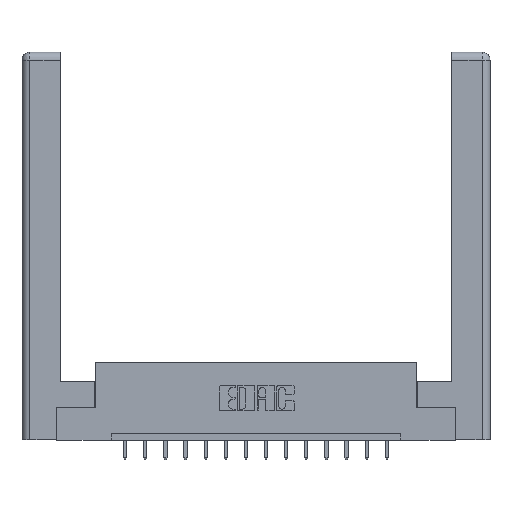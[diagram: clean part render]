
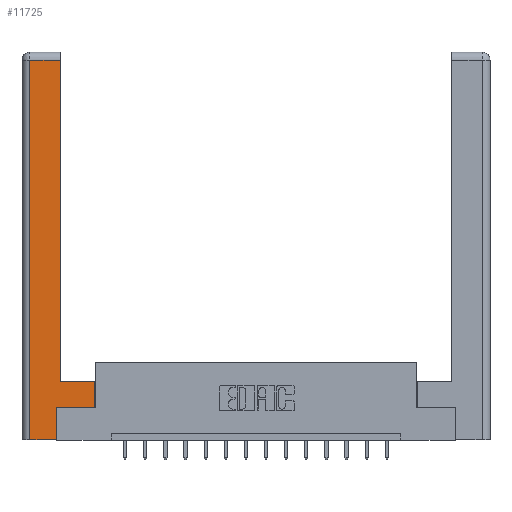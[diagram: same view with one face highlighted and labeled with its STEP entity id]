
A CAD part, top view. The second image highlights one B-rep face of the part: STEP entity #11725.
In plain terms, the highlighted planar face has unit normal (0, 0, 1).
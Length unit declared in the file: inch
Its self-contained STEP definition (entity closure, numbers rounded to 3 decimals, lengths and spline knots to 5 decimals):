
#19 = VERTEX_POINT ( 'NONE', #4875 ) ;
#131 = CARTESIAN_POINT ( 'NONE',  ( 0.565, 0.245, 0. ) ) ;
#334 = LINE ( 'NONE', #12084, #5798 ) ;
#569 = VECTOR ( 'NONE', #2073, 39.37008 ) ;
#601 = CARTESIAN_POINT ( 'NONE',  ( 0.265, 0.245, 0. ) ) ;
#858 = LINE ( 'NONE', #10067, #3469 ) ;
#895 = LINE ( 'NONE', #13281, #13758 ) ;
#1614 = DIRECTION ( 'NONE',  ( -1., 0., 0. ) ) ;
#1760 = DIRECTION ( 'NONE',  ( 0., -1., 0. ) ) ;
#1842 = DIRECTION ( 'NONE',  ( -1., 0., 0. ) ) ;
#1939 = ORIENTED_EDGE ( 'NONE', *, *, #5358, .T. ) ;
#2073 = DIRECTION ( 'NONE',  ( 0., 1., 0. ) ) ;
#2627 = LINE ( 'NONE', #14973, #569 ) ;
#2726 = VERTEX_POINT ( 'NONE', #131 ) ;
#2867 = VERTEX_POINT ( 'NONE', #6008 ) ;
#3208 = VECTOR ( 'NONE', #8772, 39.37008 ) ;
#3444 = FACE_OUTER_BOUND ( 'NONE', #5556, .T. ) ;
#3469 = VECTOR ( 'NONE', #7546, 39.37008 ) ;
#3983 = CARTESIAN_POINT ( 'NONE',  ( 0.265, 0., 0. ) ) ;
#3995 = DIRECTION ( 'NONE',  ( 1., 0., 0. ) ) ;
#4146 = CARTESIAN_POINT ( 'NONE',  ( 0.565, 0.45, 0. ) ) ;
#4260 = CARTESIAN_POINT ( 'NONE',  ( 0., 0., 0. ) ) ;
#4823 = VERTEX_POINT ( 'NONE', #12168 ) ;
#4875 = CARTESIAN_POINT ( 'NONE',  ( 0.0615, 0., 0. ) ) ;
#5358 = EDGE_CURVE ( 'NONE', #2867, #4823, #13303, .T. ) ;
#5442 = DIRECTION ( 'NONE',  ( 0., 0., -1. ) ) ;
#5556 = EDGE_LOOP ( 'NONE', ( #1939, #8867, #14191, #10448, #5648, #11729, #11336, #6467 ) ) ;
#5648 = ORIENTED_EDGE ( 'NONE', *, *, #14777, .T. ) ;
#5798 = VECTOR ( 'NONE', #1842, 39.37008 ) ;
#5878 = DIRECTION ( 'NONE',  ( 0., 1., 0. ) ) ;
#5955 = VERTEX_POINT ( 'NONE', #601 ) ;
#6008 = CARTESIAN_POINT ( 'NONE',  ( 0.295, 0.45, 0. ) ) ;
#6306 = EDGE_CURVE ( 'NONE', #8891, #2867, #9254, .T. ) ;
#6467 = ORIENTED_EDGE ( 'NONE', *, *, #6306, .T. ) ;
#6487 = VECTOR ( 'NONE', #5878, 39.37008 ) ;
#7470 = CARTESIAN_POINT ( 'NONE',  ( 0.265, 0.245, 0. ) ) ;
#7546 = DIRECTION ( 'NONE',  ( 1., 0., 0. ) ) ;
#8548 = VECTOR ( 'NONE', #16524, 39.37008 ) ;
#8772 = DIRECTION ( 'NONE',  ( -1., 0., 0. ) ) ;
#8867 = ORIENTED_EDGE ( 'NONE', *, *, #13574, .T. ) ;
#8891 = VERTEX_POINT ( 'NONE', #4146 ) ;
#9254 = LINE ( 'NONE', #11508, #3208 ) ;
#9501 = AXIS2_PLACEMENT_3D ( 'NONE', #4260, #5442, #1614 ) ;
#9997 = CARTESIAN_POINT ( 'NONE',  ( 0.0615, 2.94, 0. ) ) ;
#10000 = EDGE_CURVE ( 'NONE', #19, #11683, #12151, .T. ) ;
#10067 = CARTESIAN_POINT ( 'NONE',  ( 0.565, 0.245, 0. ) ) ;
#10384 = EDGE_CURVE ( 'NONE', #2726, #8891, #2627, .T. ) ;
#10448 = ORIENTED_EDGE ( 'NONE', *, *, #10000, .T. ) ;
#10533 = EDGE_CURVE ( 'NONE', #5955, #2726, #858, .T. ) ;
#11103 = CARTESIAN_POINT ( 'NONE',  ( 0.295, 3., 0. ) ) ;
#11336 = ORIENTED_EDGE ( 'NONE', *, *, #10384, .T. ) ;
#11508 = CARTESIAN_POINT ( 'NONE',  ( 0.295, 0.45, 0. ) ) ;
#11683 = VERTEX_POINT ( 'NONE', #3983 ) ;
#11725 = ADVANCED_FACE ( 'NONE', ( #3444 ), #12759, .F. ) ;
#11729 = ORIENTED_EDGE ( 'NONE', *, *, #10533, .T. ) ;
#12084 = CARTESIAN_POINT ( 'NONE',  ( 0.0615, 2.94, 0. ) ) ;
#12151 = LINE ( 'NONE', #14283, #16004 ) ;
#12168 = CARTESIAN_POINT ( 'NONE',  ( 0.295, 2.94, 0. ) ) ;
#12759 = PLANE ( 'NONE',  #9501 ) ;
#13281 = CARTESIAN_POINT ( 'NONE',  ( 0.0615, 0., 0. ) ) ;
#13303 = LINE ( 'NONE', #11103, #6487 ) ;
#13574 = EDGE_CURVE ( 'NONE', #4823, #14771, #334, .T. ) ;
#13758 = VECTOR ( 'NONE', #1760, 39.37008 ) ;
#14191 = ORIENTED_EDGE ( 'NONE', *, *, #15306, .T. ) ;
#14283 = CARTESIAN_POINT ( 'NONE',  ( 0.265, 0., 0. ) ) ;
#14771 = VERTEX_POINT ( 'NONE', #9997 ) ;
#14777 = EDGE_CURVE ( 'NONE', #11683, #5955, #15813, .T. ) ;
#14973 = CARTESIAN_POINT ( 'NONE',  ( 0.565, 0.45, 0. ) ) ;
#15306 = EDGE_CURVE ( 'NONE', #14771, #19, #895, .T. ) ;
#15813 = LINE ( 'NONE', #7470, #8548 ) ;
#16004 = VECTOR ( 'NONE', #3995, 39.37008 ) ;
#16524 = DIRECTION ( 'NONE',  ( 0., 1., 0. ) ) ;
